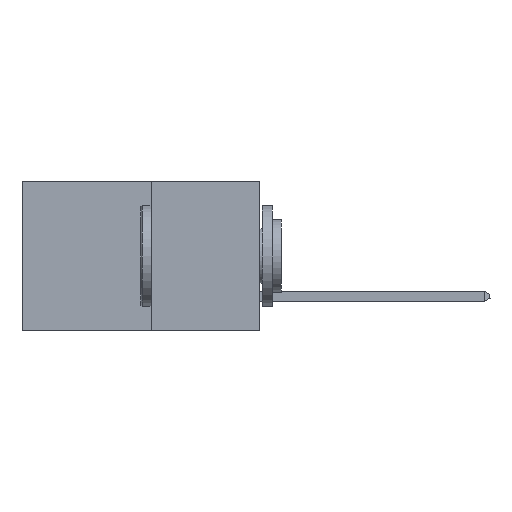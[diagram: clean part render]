
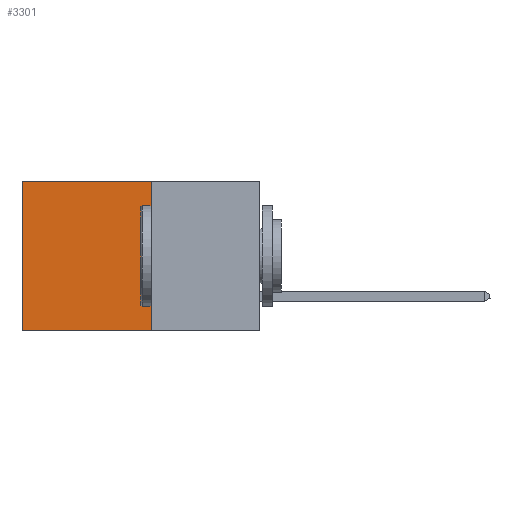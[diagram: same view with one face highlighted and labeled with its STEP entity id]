
A CAD part, left-side view. The second image highlights one B-rep face of the part: STEP entity #3301.
In plain terms, the highlighted planar face has unit normal (-1, 0, 0).
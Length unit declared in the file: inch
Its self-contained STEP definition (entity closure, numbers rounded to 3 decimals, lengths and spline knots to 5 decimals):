
#678 = AXIS2_PLACEMENT_3D ( 'NONE', #6353, #11526, #2386 ) ;
#954 = CARTESIAN_POINT ( 'NONE',  ( 0.277, 0.27, 0. ) ) ;
#1065 = CARTESIAN_POINT ( 'NONE',  ( 0.277, 0.27, -0.37 ) ) ;
#1294 = VECTOR ( 'NONE', #5528, 39.37008 ) ;
#1378 = DIRECTION ( 'NONE',  ( 0., 1., 0. ) ) ;
#1384 = EDGE_CURVE ( 'NONE', #8685, #4919, #2963, .T. ) ;
#1597 = ORIENTED_EDGE ( 'NONE', *, *, #1384, .F. ) ;
#2386 = DIRECTION ( 'NONE',  ( 0., 0., -1. ) ) ;
#2423 = ORIENTED_EDGE ( 'NONE', *, *, #7028, .T. ) ;
#2535 = VECTOR ( 'NONE', #6092, 39.37008 ) ;
#2670 = VERTEX_POINT ( 'NONE', #10049 ) ;
#2872 = LINE ( 'NONE', #5138, #2535 ) ;
#2963 = LINE ( 'NONE', #1065, #5564 ) ;
#3301 = ADVANCED_FACE ( 'NONE', ( #11284 ), #4623, .F. ) ;
#3485 = EDGE_CURVE ( 'NONE', #6743, #8685, #11728, .T. ) ;
#4623 = PLANE ( 'NONE',  #678 ) ;
#4919 = VERTEX_POINT ( 'NONE', #7203 ) ;
#5138 = CARTESIAN_POINT ( 'NONE',  ( 0.277, 0.59, -0.37 ) ) ;
#5528 = DIRECTION ( 'NONE',  ( 0., 0., -1. ) ) ;
#5564 = VECTOR ( 'NONE', #1378, 39.37008 ) ;
#5954 = ORIENTED_EDGE ( 'NONE', *, *, #7255, .T. ) ;
#6092 = DIRECTION ( 'NONE',  ( 0., 0., -1. ) ) ;
#6353 = CARTESIAN_POINT ( 'NONE',  ( 0.277, 0.27, -0.37 ) ) ;
#6558 = EDGE_LOOP ( 'NONE', ( #5954, #1597, #11574, #2423 ) ) ;
#6743 = VERTEX_POINT ( 'NONE', #954 ) ;
#7028 = EDGE_CURVE ( 'NONE', #6743, #2670, #9881, .T. ) ;
#7203 = CARTESIAN_POINT ( 'NONE',  ( 0.277, 0.59, -0.37 ) ) ;
#7255 = EDGE_CURVE ( 'NONE', #2670, #4919, #2872, .T. ) ;
#7261 = VECTOR ( 'NONE', #11561, 39.37008 ) ;
#8685 = VERTEX_POINT ( 'NONE', #12175 ) ;
#9881 = LINE ( 'NONE', #12488, #7261 ) ;
#10049 = CARTESIAN_POINT ( 'NONE',  ( 0.277, 0.59, 0. ) ) ;
#10700 = CARTESIAN_POINT ( 'NONE',  ( 0.277, 0.27, -0.37 ) ) ;
#11284 = FACE_OUTER_BOUND ( 'NONE', #6558, .T. ) ;
#11526 = DIRECTION ( 'NONE',  ( 1., 0., 0. ) ) ;
#11561 = DIRECTION ( 'NONE',  ( 0., 1., 0. ) ) ;
#11574 = ORIENTED_EDGE ( 'NONE', *, *, #3485, .F. ) ;
#11728 = LINE ( 'NONE', #10700, #1294 ) ;
#12175 = CARTESIAN_POINT ( 'NONE',  ( 0.277, 0.27, -0.37 ) ) ;
#12488 = CARTESIAN_POINT ( 'NONE',  ( 0.277, 0.27, 0. ) ) ;
